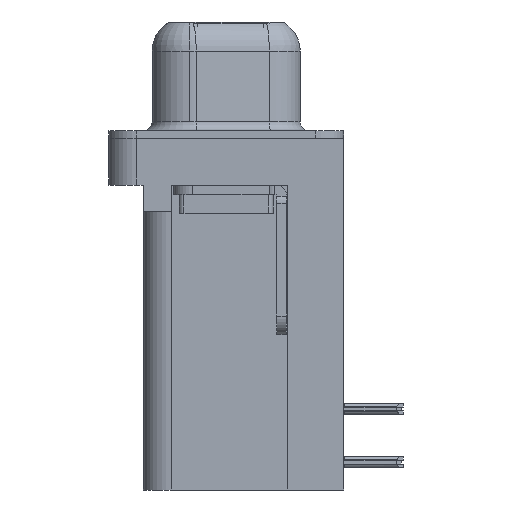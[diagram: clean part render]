
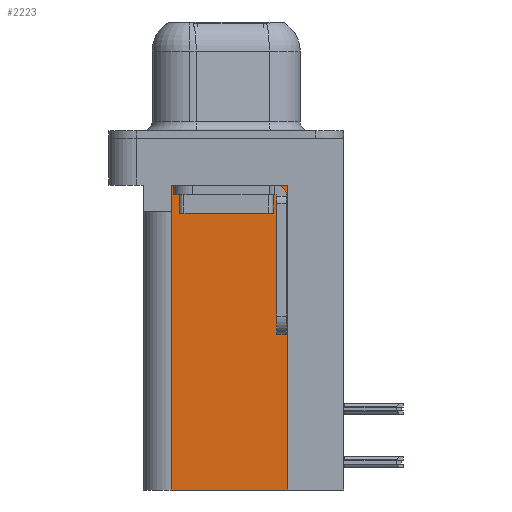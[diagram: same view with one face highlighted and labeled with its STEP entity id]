
A CAD part, left-side view. The second image highlights one B-rep face of the part: STEP entity #2223.
In plain terms, the highlighted planar face has unit normal (-1, 0, 0).
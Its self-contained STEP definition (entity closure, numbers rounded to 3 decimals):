
#350 = VECTOR ( 'NONE', #28451, 1000. ) ;
#541 = LINE ( 'NONE', #7336, #350 ) ;
#1358 = VERTEX_POINT ( 'NONE', #25989 ) ;
#2223 = ADVANCED_FACE ( 'NONE', ( #4553 ), #23816, .F. ) ;
#4003 = ORIENTED_EDGE ( 'NONE', *, *, #8164, .T. ) ;
#4314 = VERTEX_POINT ( 'NONE', #23315 ) ;
#4456 = DIRECTION ( 'NONE',  ( 0., 1., 0. ) ) ;
#4553 = FACE_OUTER_BOUND ( 'NONE', #28432, .T. ) ;
#7010 = VECTOR ( 'NONE', #4456, 1000. ) ;
#7185 = CARTESIAN_POINT ( 'NONE',  ( 3.79, -3.295, -18.76 ) ) ;
#7277 = LINE ( 'NONE', #33290, #7010 ) ;
#7336 = CARTESIAN_POINT ( 'NONE',  ( 3.79, 0., -3.9 ) ) ;
#8164 = EDGE_CURVE ( 'NONE', #31959, #23917, #10029, .T. ) ;
#9397 = VECTOR ( 'NONE', #13406, 1000. ) ;
#9908 = EDGE_CURVE ( 'NONE', #23917, #24636, #541, .T. ) ;
#10029 = LINE ( 'NONE', #10742, #9397 ) ;
#10742 = CARTESIAN_POINT ( 'NONE',  ( 3.79, 2.895, -3.9 ) ) ;
#12737 = CARTESIAN_POINT ( 'NONE',  ( 3.79, 2.895, -2.5 ) ) ;
#13406 = DIRECTION ( 'NONE',  ( 0., 0., -1. ) ) ;
#14379 = AXIS2_PLACEMENT_3D ( 'NONE', #23768, #20309, #20031 ) ;
#15186 = ORIENTED_EDGE ( 'NONE', *, *, #19051, .T. ) ;
#15368 = EDGE_CURVE ( 'NONE', #22354, #24636, #28064, .T. ) ;
#16126 = EDGE_CURVE ( 'NONE', #4314, #1358, #23666, .T. ) ;
#16426 = EDGE_CURVE ( 'NONE', #4314, #22354, #22276, .T. ) ;
#17250 = ORIENTED_EDGE ( 'NONE', *, *, #9908, .T. ) ;
#17630 = DIRECTION ( 'NONE',  ( 0., 1., 0. ) ) ;
#18968 = DIRECTION ( 'NONE',  ( 0., 0., 1. ) ) ;
#19051 = EDGE_CURVE ( 'NONE', #1358, #31959, #7277, .T. ) ;
#20031 = DIRECTION ( 'NONE',  ( 0., 1., 0. ) ) ;
#20309 = DIRECTION ( 'NONE',  ( 1., 0., 0. ) ) ;
#22276 = LINE ( 'NONE', #7185, #22417 ) ;
#22354 = VERTEX_POINT ( 'NONE', #26663 ) ;
#22417 = VECTOR ( 'NONE', #17630, 1000. ) ;
#23315 = CARTESIAN_POINT ( 'NONE',  ( 3.79, -3.295, -18.76 ) ) ;
#23666 = LINE ( 'NONE', #24200, #23820 ) ;
#23768 = CARTESIAN_POINT ( 'NONE',  ( 3.79, -3.295, -18.76 ) ) ;
#23816 = PLANE ( 'NONE',  #14379 ) ;
#23820 = VECTOR ( 'NONE', #18968, 1000. ) ;
#23917 = VERTEX_POINT ( 'NONE', #32970 ) ;
#24200 = CARTESIAN_POINT ( 'NONE',  ( 3.79, -3.295, -18.76 ) ) ;
#24636 = VERTEX_POINT ( 'NONE', #33044 ) ;
#25981 = CARTESIAN_POINT ( 'NONE',  ( 3.79, 2.925, -18.76 ) ) ;
#25989 = CARTESIAN_POINT ( 'NONE',  ( 3.79, -3.295, -2.5 ) ) ;
#26663 = CARTESIAN_POINT ( 'NONE',  ( 3.79, 2.925, -18.76 ) ) ;
#26920 = ORIENTED_EDGE ( 'NONE', *, *, #16426, .F. ) ;
#27945 = VECTOR ( 'NONE', #31249, 1000. ) ;
#28064 = LINE ( 'NONE', #25981, #27945 ) ;
#28117 = ORIENTED_EDGE ( 'NONE', *, *, #16126, .T. ) ;
#28432 = EDGE_LOOP ( 'NONE', ( #15186, #4003, #17250, #33492, #26920, #28117 ) ) ;
#28451 = DIRECTION ( 'NONE',  ( 0., 1., 0. ) ) ;
#31249 = DIRECTION ( 'NONE',  ( 0., 0., 1. ) ) ;
#31959 = VERTEX_POINT ( 'NONE', #12737 ) ;
#32970 = CARTESIAN_POINT ( 'NONE',  ( 3.79, 2.895, -3.9 ) ) ;
#33044 = CARTESIAN_POINT ( 'NONE',  ( 3.79, 2.925, -3.9 ) ) ;
#33290 = CARTESIAN_POINT ( 'NONE',  ( 3.79, -3.295, -2.5 ) ) ;
#33492 = ORIENTED_EDGE ( 'NONE', *, *, #15368, .F. ) ;
